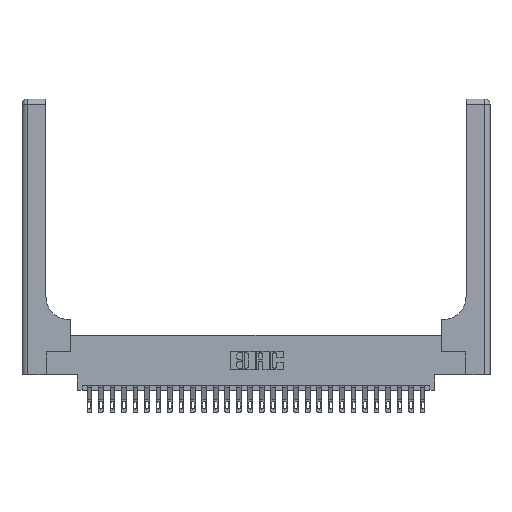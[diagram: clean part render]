
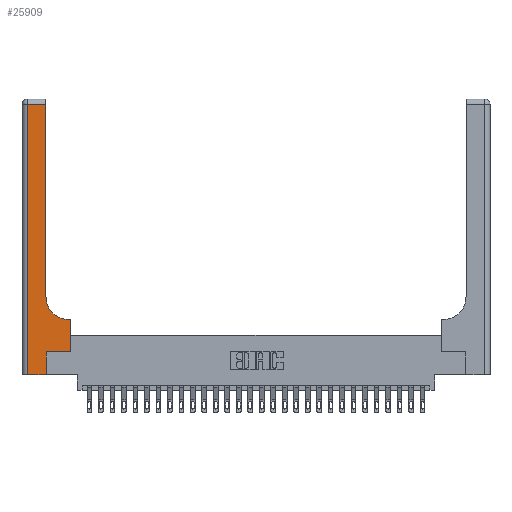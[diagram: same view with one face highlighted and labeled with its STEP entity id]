
A CAD part, top view. The second image highlights one B-rep face of the part: STEP entity #25909.
In plain terms, the highlighted planar face has unit normal (0, 0, 1).
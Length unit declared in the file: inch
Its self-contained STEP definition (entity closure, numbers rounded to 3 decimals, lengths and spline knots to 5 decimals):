
#552 = CARTESIAN_POINT ( 'NONE',  ( 0.265, 0., 0.37 ) ) ;
#1023 = LINE ( 'NONE', #20359, #17070 ) ;
#1260 = ORIENTED_EDGE ( 'NONE', *, *, #18601, .T. ) ;
#1262 = CARTESIAN_POINT ( 'NONE',  ( 0.06, 0., 0.37 ) ) ;
#1498 = DIRECTION ( 'NONE',  ( -1., 0., 0. ) ) ;
#2544 = VECTOR ( 'NONE', #10642, 39.37008 ) ;
#2613 = LINE ( 'NONE', #6826, #24048 ) ;
#2820 = CARTESIAN_POINT ( 'NONE',  ( 0.528, 0.6, 0.37 ) ) ;
#2880 = CARTESIAN_POINT ( 'NONE',  ( 0.51, 0.85, 0.37 ) ) ;
#3713 = VERTEX_POINT ( 'NONE', #17006 ) ;
#3773 = EDGE_CURVE ( 'NONE', #3713, #10437, #23939, .T. ) ;
#4106 = CARTESIAN_POINT ( 'NONE',  ( 0.06, 2.94, 0.37 ) ) ;
#4532 = ORIENTED_EDGE ( 'NONE', *, *, #4752, .T. ) ;
#4752 = EDGE_CURVE ( 'NONE', #6567, #6841, #13611, .T. ) ;
#4959 = DIRECTION ( 'NONE',  ( 1., 0., 0. ) ) ;
#5127 = VERTEX_POINT ( 'NONE', #12900 ) ;
#5782 = VERTEX_POINT ( 'NONE', #21360 ) ;
#6167 = ORIENTED_EDGE ( 'NONE', *, *, #8692, .T. ) ;
#6567 = VERTEX_POINT ( 'NONE', #2820 ) ;
#6826 = CARTESIAN_POINT ( 'NONE',  ( 0.26, 3., 0.37 ) ) ;
#6841 = VERTEX_POINT ( 'NONE', #14082 ) ;
#6845 = ORIENTED_EDGE ( 'NONE', *, *, #11991, .T. ) ;
#6941 = CARTESIAN_POINT ( 'NONE',  ( 0.265, 0.25, 0.37 ) ) ;
#7230 = EDGE_LOOP ( 'NONE', ( #6167, #11791, #1260, #6845, #13104, #24025, #8844, #4532, #15695 ) ) ;
#7899 = DIRECTION ( 'NONE',  ( 1., 0., 0. ) ) ;
#7918 = VECTOR ( 'NONE', #19819, 39.37008 ) ;
#8083 = VECTOR ( 'NONE', #15222, 39.37008 ) ;
#8578 = LINE ( 'NONE', #9469, #7918 ) ;
#8692 = EDGE_CURVE ( 'NONE', #5127, #5782, #2613, .T. ) ;
#8844 = ORIENTED_EDGE ( 'NONE', *, *, #26135, .T. ) ;
#9469 = CARTESIAN_POINT ( 'NONE',  ( 0., 0., 0.37 ) ) ;
#9632 = CARTESIAN_POINT ( 'NONE',  ( 0.26, 0.6, 0.37 ) ) ;
#10437 = VERTEX_POINT ( 'NONE', #6941 ) ;
#10642 = DIRECTION ( 'NONE',  ( -1., 0., 0. ) ) ;
#11791 = ORIENTED_EDGE ( 'NONE', *, *, #20007, .T. ) ;
#11827 = CARTESIAN_POINT ( 'NONE',  ( 0.06, 3., 0.37 ) ) ;
#11912 = FACE_OUTER_BOUND ( 'NONE', #7230, .T. ) ;
#11980 = PLANE ( 'NONE',  #22010 ) ;
#11991 = EDGE_CURVE ( 'NONE', #19745, #3713, #8578, .T. ) ;
#12880 = LINE ( 'NONE', #23320, #17718 ) ;
#12900 = CARTESIAN_POINT ( 'NONE',  ( 0.26, 0.85, 0.37 ) ) ;
#13104 = ORIENTED_EDGE ( 'NONE', *, *, #3773, .T. ) ;
#13611 = LINE ( 'NONE', #9632, #20402 ) ;
#13925 = DIRECTION ( 'NONE',  ( 0., -1., 0. ) ) ;
#14068 = DIRECTION ( 'NONE',  ( 0., 0., -1. ) ) ;
#14082 = CARTESIAN_POINT ( 'NONE',  ( 0.51, 0.6, 0.37 ) ) ;
#14349 = LINE ( 'NONE', #22996, #2544 ) ;
#15222 = DIRECTION ( 'NONE',  ( 0., 1., 0. ) ) ;
#15695 = ORIENTED_EDGE ( 'NONE', *, *, #17232, .T. ) ;
#17006 = CARTESIAN_POINT ( 'NONE',  ( 0.265, 0., 0.37 ) ) ;
#17070 = VECTOR ( 'NONE', #7899, 39.37008 ) ;
#17232 = EDGE_CURVE ( 'NONE', #6841, #5127, #21867, .T. ) ;
#17501 = DIRECTION ( 'NONE',  ( 0., 0., -1. ) ) ;
#17589 = VECTOR ( 'NONE', #13925, 39.37008 ) ;
#17718 = VECTOR ( 'NONE', #25334, 39.37008 ) ;
#18240 = LINE ( 'NONE', #11827, #17589 ) ;
#18601 = EDGE_CURVE ( 'NONE', #23345, #19745, #18240, .T. ) ;
#19745 = VERTEX_POINT ( 'NONE', #1262 ) ;
#19819 = DIRECTION ( 'NONE',  ( 1., 0., 0. ) ) ;
#20007 = EDGE_CURVE ( 'NONE', #5782, #23345, #14349, .T. ) ;
#20359 = CARTESIAN_POINT ( 'NONE',  ( 0.265, 0.25, 0.37 ) ) ;
#20402 = VECTOR ( 'NONE', #24058, 39.37008 ) ;
#20403 = AXIS2_PLACEMENT_3D ( 'NONE', #2880, #17501, #4959 ) ;
#21360 = CARTESIAN_POINT ( 'NONE',  ( 0.26, 2.94, 0.37 ) ) ;
#21481 = DIRECTION ( 'NONE',  ( 0., 1., 0. ) ) ;
#21551 = VERTEX_POINT ( 'NONE', #25755 ) ;
#21867 = CIRCLE ( 'NONE', #20403, 0.25 ) ;
#22010 = AXIS2_PLACEMENT_3D ( 'NONE', #24285, #14068, #1498 ) ;
#22996 = CARTESIAN_POINT ( 'NONE',  ( 0., 2.94, 0.37 ) ) ;
#23235 = EDGE_CURVE ( 'NONE', #10437, #21551, #1023, .T. ) ;
#23320 = CARTESIAN_POINT ( 'NONE',  ( 0.528, 0.25, 0.37 ) ) ;
#23345 = VERTEX_POINT ( 'NONE', #4106 ) ;
#23939 = LINE ( 'NONE', #552, #8083 ) ;
#24025 = ORIENTED_EDGE ( 'NONE', *, *, #23235, .T. ) ;
#24048 = VECTOR ( 'NONE', #21481, 39.37008 ) ;
#24058 = DIRECTION ( 'NONE',  ( -1., 0., 0. ) ) ;
#24285 = CARTESIAN_POINT ( 'NONE',  ( 0., 3., 0.37 ) ) ;
#25334 = DIRECTION ( 'NONE',  ( 0., 1., 0. ) ) ;
#25755 = CARTESIAN_POINT ( 'NONE',  ( 0.528, 0.25, 0.37 ) ) ;
#25909 = ADVANCED_FACE ( 'NONE', ( #11912 ), #11980, .F. ) ;
#26135 = EDGE_CURVE ( 'NONE', #21551, #6567, #12880, .T. ) ;
